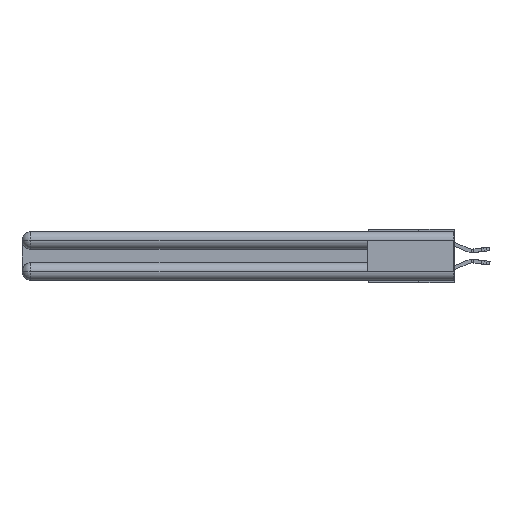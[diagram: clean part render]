
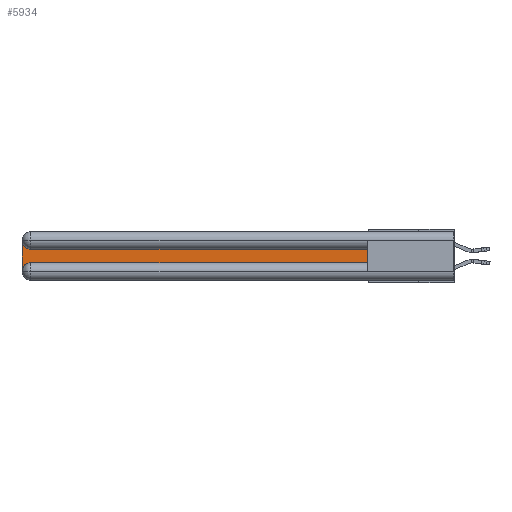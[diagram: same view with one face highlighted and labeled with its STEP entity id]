
A CAD part, left-side view. The second image highlights one B-rep face of the part: STEP entity #5934.
In plain terms, the highlighted planar face has unit normal (-1, 0, 0).
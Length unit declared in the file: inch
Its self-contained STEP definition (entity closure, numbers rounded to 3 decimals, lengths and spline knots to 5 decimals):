
#220 = VECTOR ( 'NONE', #12711, 39.37008 ) ;
#285 = EDGE_CURVE ( 'NONE', #15132, #17899, #10299, .T. ) ;
#467 = CARTESIAN_POINT ( 'NONE',  ( 0.075, 3., -0.2175 ) ) ;
#1755 = DIRECTION ( 'NONE',  ( 0., -1., 0. ) ) ;
#2292 = CARTESIAN_POINT ( 'NONE',  ( 0.075, 2.94, -0.2775 ) ) ;
#2383 = CARTESIAN_POINT ( 'NONE',  ( 0.075, 0.6, -0.2175 ) ) ;
#2505 = DIRECTION ( 'NONE',  ( 1., 0., 0. ) ) ;
#3107 = FACE_OUTER_BOUND ( 'NONE', #24205, .T. ) ;
#3149 = DIRECTION ( 'NONE',  ( 0., 0., -1. ) ) ;
#3328 = LINE ( 'NONE', #14346, #16063 ) ;
#4223 = CARTESIAN_POINT ( 'NONE',  ( 0.075, 2.94, -0.0625 ) ) ;
#4972 = CARTESIAN_POINT ( 'NONE',  ( 0.075, 2.94, -0.1225 ) ) ;
#5098 = ORIENTED_EDGE ( 'NONE', *, *, #20421, .T. ) ;
#5193 = PLANE ( 'NONE',  #8582 ) ;
#5546 = AXIS2_PLACEMENT_3D ( 'NONE', #2292, #2505, #7608 ) ;
#5934 = ADVANCED_FACE ( 'NONE', ( #3107 ), #5193, .F. ) ;
#5980 = ORIENTED_EDGE ( 'NONE', *, *, #19942, .T. ) ;
#6571 = DIRECTION ( 'NONE',  ( 1., 0., 0. ) ) ;
#7608 = DIRECTION ( 'NONE',  ( 0., 0., -1. ) ) ;
#8582 = AXIS2_PLACEMENT_3D ( 'NONE', #20196, #20539, #17963 ) ;
#9344 = VECTOR ( 'NONE', #3149, 39.37008 ) ;
#10299 = LINE ( 'NONE', #19612, #16317 ) ;
#10592 = VERTEX_POINT ( 'NONE', #27561 ) ;
#10872 = ORIENTED_EDGE ( 'NONE', *, *, #11143, .T. ) ;
#11143 = EDGE_CURVE ( 'NONE', #10592, #23103, #26877, .T. ) ;
#12711 = DIRECTION ( 'NONE',  ( 0., 0., 1. ) ) ;
#12745 = CARTESIAN_POINT ( 'NONE',  ( 0.075, 2.94, -0.2175 ) ) ;
#13371 = ORIENTED_EDGE ( 'NONE', *, *, #285, .T. ) ;
#14346 = CARTESIAN_POINT ( 'NONE',  ( 0.075, 0.6, -0.2175 ) ) ;
#15132 = VERTEX_POINT ( 'NONE', #20373 ) ;
#15760 = AXIS2_PLACEMENT_3D ( 'NONE', #4223, #6571, #26710 ) ;
#16063 = VECTOR ( 'NONE', #1755, 39.37008 ) ;
#16317 = VECTOR ( 'NONE', #17261, 39.37008 ) ;
#17261 = DIRECTION ( 'NONE',  ( 0., 1., 0. ) ) ;
#17899 = VERTEX_POINT ( 'NONE', #4972 ) ;
#17963 = DIRECTION ( 'NONE',  ( 0., 0., -1. ) ) ;
#18919 = LINE ( 'NONE', #2383, #220 ) ;
#19342 = EDGE_CURVE ( 'NONE', #27997, #27536, #3328, .T. ) ;
#19612 = CARTESIAN_POINT ( 'NONE',  ( 0.075, 0.6, -0.1225 ) ) ;
#19942 = EDGE_CURVE ( 'NONE', #23103, #27997, #19979, .T. ) ;
#19979 = CIRCLE ( 'NONE', #5546, 0.06 ) ;
#20196 = CARTESIAN_POINT ( 'NONE',  ( 0.075, 3., -0.1225 ) ) ;
#20373 = CARTESIAN_POINT ( 'NONE',  ( 0.075, 0.6, -0.1225 ) ) ;
#20421 = EDGE_CURVE ( 'NONE', #17899, #10592, #26728, .T. ) ;
#20539 = DIRECTION ( 'NONE',  ( 1., 0., 0. ) ) ;
#22311 = CARTESIAN_POINT ( 'NONE',  ( 0.075, 0.6, -0.2175 ) ) ;
#22759 = CARTESIAN_POINT ( 'NONE',  ( 0.075, 3., -0.2775 ) ) ;
#22769 = ORIENTED_EDGE ( 'NONE', *, *, #23536, .T. ) ;
#23103 = VERTEX_POINT ( 'NONE', #22759 ) ;
#23536 = EDGE_CURVE ( 'NONE', #27536, #15132, #18919, .T. ) ;
#24205 = EDGE_LOOP ( 'NONE', ( #13371, #5098, #10872, #5980, #26542, #22769 ) ) ;
#26542 = ORIENTED_EDGE ( 'NONE', *, *, #19342, .T. ) ;
#26710 = DIRECTION ( 'NONE',  ( 0., 0., -1. ) ) ;
#26728 = CIRCLE ( 'NONE', #15760, 0.06 ) ;
#26877 = LINE ( 'NONE', #467, #9344 ) ;
#27536 = VERTEX_POINT ( 'NONE', #22311 ) ;
#27561 = CARTESIAN_POINT ( 'NONE',  ( 0.075, 3., -0.0625 ) ) ;
#27997 = VERTEX_POINT ( 'NONE', #12745 ) ;
